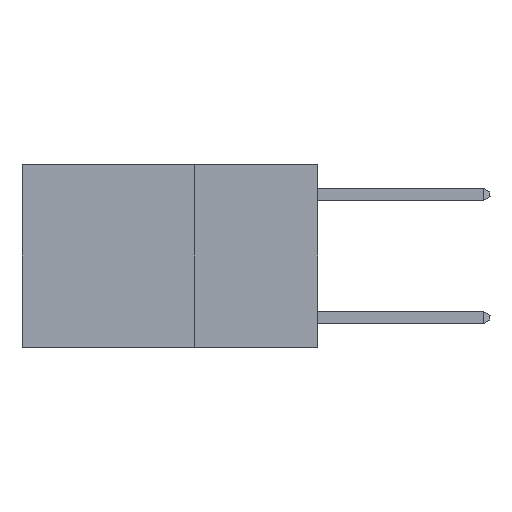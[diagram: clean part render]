
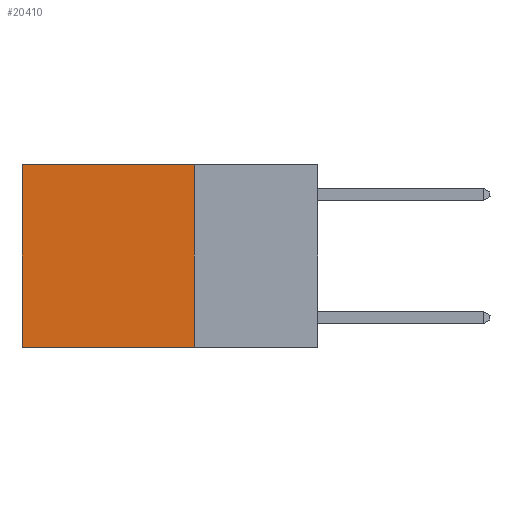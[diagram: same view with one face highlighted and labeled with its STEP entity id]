
A CAD part, left-side view. The second image highlights one B-rep face of the part: STEP entity #20410.
In plain terms, the highlighted planar face has unit normal (-1, 0, 0).
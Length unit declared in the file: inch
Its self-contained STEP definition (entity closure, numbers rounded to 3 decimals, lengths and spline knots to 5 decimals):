
#400 = VERTEX_POINT ( 'NONE', #14841 ) ;
#742 = CARTESIAN_POINT ( 'NONE',  ( 0.2625, 0.25, 0. ) ) ;
#1442 = EDGE_CURVE ( 'NONE', #26573, #400, #7327, .T. ) ;
#4431 = ORIENTED_EDGE ( 'NONE', *, *, #10748, .F. ) ;
#5021 = CARTESIAN_POINT ( 'NONE',  ( 0.2625, 0.25, -0.37 ) ) ;
#7103 = LINE ( 'NONE', #15581, #19071 ) ;
#7327 = LINE ( 'NONE', #16244, #26111 ) ;
#7473 = DIRECTION ( 'NONE',  ( 0., 0., -1. ) ) ;
#10748 = EDGE_CURVE ( 'NONE', #26840, #21616, #21434, .T. ) ;
#11097 = EDGE_CURVE ( 'NONE', #26840, #26573, #7103, .T. ) ;
#11952 = DIRECTION ( 'NONE',  ( 0., 0., -1. ) ) ;
#12104 = VECTOR ( 'NONE', #17356, 39.37008 ) ;
#14841 = CARTESIAN_POINT ( 'NONE',  ( 0.2625, 0.6, -0.37 ) ) ;
#15581 = CARTESIAN_POINT ( 'NONE',  ( 0.2625, 0.25, 0. ) ) ;
#16244 = CARTESIAN_POINT ( 'NONE',  ( 0.2625, 0.6, 0. ) ) ;
#17356 = DIRECTION ( 'NONE',  ( 0., 1., 0. ) ) ;
#18904 = DIRECTION ( 'NONE',  ( 1., 0., 0. ) ) ;
#19071 = VECTOR ( 'NONE', #22607, 39.37008 ) ;
#20410 = ADVANCED_FACE ( 'NONE', ( #25643 ), #21240, .F. ) ;
#20430 = ORIENTED_EDGE ( 'NONE', *, *, #1442, .T. ) ;
#21174 = ORIENTED_EDGE ( 'NONE', *, *, #22761, .F. ) ;
#21240 = PLANE ( 'NONE',  #27331 ) ;
#21434 = LINE ( 'NONE', #25425, #27479 ) ;
#21616 = VERTEX_POINT ( 'NONE', #5021 ) ;
#22607 = DIRECTION ( 'NONE',  ( 0., 1., 0. ) ) ;
#22761 = EDGE_CURVE ( 'NONE', #21616, #400, #23804, .T. ) ;
#23010 = DIRECTION ( 'NONE',  ( 0., 0., -1. ) ) ;
#23804 = LINE ( 'NONE', #25733, #12104 ) ;
#24773 = CARTESIAN_POINT ( 'NONE',  ( 0.2625, 0.6, 0. ) ) ;
#25425 = CARTESIAN_POINT ( 'NONE',  ( 0.2625, 0.25, 0. ) ) ;
#25643 = FACE_OUTER_BOUND ( 'NONE', #26274, .T. ) ;
#25733 = CARTESIAN_POINT ( 'NONE',  ( 0.2625, 0.25, -0.37 ) ) ;
#26111 = VECTOR ( 'NONE', #7473, 39.37008 ) ;
#26274 = EDGE_LOOP ( 'NONE', ( #20430, #21174, #4431, #28144 ) ) ;
#26573 = VERTEX_POINT ( 'NONE', #24773 ) ;
#26840 = VERTEX_POINT ( 'NONE', #28651 ) ;
#27331 = AXIS2_PLACEMENT_3D ( 'NONE', #742, #18904, #23010 ) ;
#27479 = VECTOR ( 'NONE', #11952, 39.37008 ) ;
#28144 = ORIENTED_EDGE ( 'NONE', *, *, #11097, .T. ) ;
#28651 = CARTESIAN_POINT ( 'NONE',  ( 0.2625, 0.25, 0. ) ) ;
